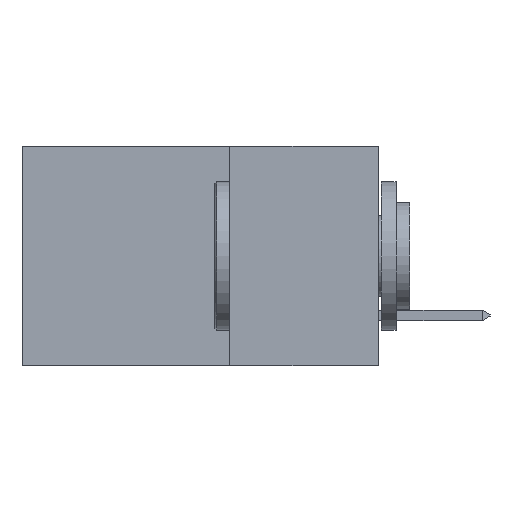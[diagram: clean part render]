
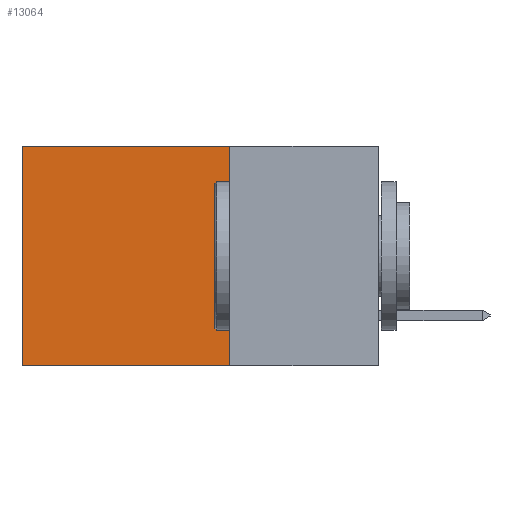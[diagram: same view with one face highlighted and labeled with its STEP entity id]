
A CAD part, left-side view. The second image highlights one B-rep face of the part: STEP entity #13064.
In plain terms, the highlighted planar face has unit normal (-1, 0, 0).
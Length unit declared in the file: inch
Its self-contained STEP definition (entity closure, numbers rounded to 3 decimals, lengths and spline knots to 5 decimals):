
#735 = DIRECTION ( 'NONE',  ( 0., 1., 0. ) ) ;
#1082 = CARTESIAN_POINT ( 'NONE',  ( 0.298, 0.6, -0.37 ) ) ;
#1161 = FACE_OUTER_BOUND ( 'NONE', #6706, .T. ) ;
#1268 = VERTEX_POINT ( 'NONE', #15560 ) ;
#1635 = EDGE_CURVE ( 'NONE', #4097, #1268, #8937, .T. ) ;
#1774 = VECTOR ( 'NONE', #2241, 39.37008 ) ;
#2192 = CARTESIAN_POINT ( 'NONE',  ( 0.298, 0.25, 0. ) ) ;
#2241 = DIRECTION ( 'NONE',  ( 0., 1., 0. ) ) ;
#2282 = CARTESIAN_POINT ( 'NONE',  ( 0.298, 0.25, 0. ) ) ;
#2602 = CARTESIAN_POINT ( 'NONE',  ( 0.298, 0.6, 0. ) ) ;
#3576 = VECTOR ( 'NONE', #9677, 39.37008 ) ;
#3855 = DIRECTION ( 'NONE',  ( 0., 0., -1. ) ) ;
#4097 = VERTEX_POINT ( 'NONE', #2282 ) ;
#5414 = VECTOR ( 'NONE', #3855, 39.37008 ) ;
#6309 = EDGE_CURVE ( 'NONE', #4097, #10080, #9425, .T. ) ;
#6706 = EDGE_LOOP ( 'NONE', ( #9684, #12220, #10862, #11093 ) ) ;
#7176 = CARTESIAN_POINT ( 'NONE',  ( 0.298, 0.25, 0. ) ) ;
#7827 = AXIS2_PLACEMENT_3D ( 'NONE', #7176, #15777, #8426 ) ;
#8426 = DIRECTION ( 'NONE',  ( 0., 0., -1. ) ) ;
#8733 = LINE ( 'NONE', #2602, #5414 ) ;
#8937 = LINE ( 'NONE', #14243, #11835 ) ;
#9085 = CARTESIAN_POINT ( 'NONE',  ( 0.298, 0.25, -0.37 ) ) ;
#9425 = LINE ( 'NONE', #2192, #3576 ) ;
#9677 = DIRECTION ( 'NONE',  ( 0., 0., -1. ) ) ;
#9684 = ORIENTED_EDGE ( 'NONE', *, *, #9925, .T. ) ;
#9925 = EDGE_CURVE ( 'NONE', #1268, #10464, #8733, .T. ) ;
#10080 = VERTEX_POINT ( 'NONE', #9085 ) ;
#10464 = VERTEX_POINT ( 'NONE', #1082 ) ;
#10862 = ORIENTED_EDGE ( 'NONE', *, *, #6309, .F. ) ;
#11093 = ORIENTED_EDGE ( 'NONE', *, *, #1635, .T. ) ;
#11318 = LINE ( 'NONE', #14609, #1774 ) ;
#11835 = VECTOR ( 'NONE', #735, 39.37008 ) ;
#12220 = ORIENTED_EDGE ( 'NONE', *, *, #15700, .F. ) ;
#13064 = ADVANCED_FACE ( 'NONE', ( #1161 ), #14580, .F. ) ;
#14243 = CARTESIAN_POINT ( 'NONE',  ( 0.298, 0.25, 0. ) ) ;
#14580 = PLANE ( 'NONE',  #7827 ) ;
#14609 = CARTESIAN_POINT ( 'NONE',  ( 0.298, 0.25, -0.37 ) ) ;
#15560 = CARTESIAN_POINT ( 'NONE',  ( 0.298, 0.6, 0. ) ) ;
#15700 = EDGE_CURVE ( 'NONE', #10080, #10464, #11318, .T. ) ;
#15777 = DIRECTION ( 'NONE',  ( 1., 0., 0. ) ) ;
